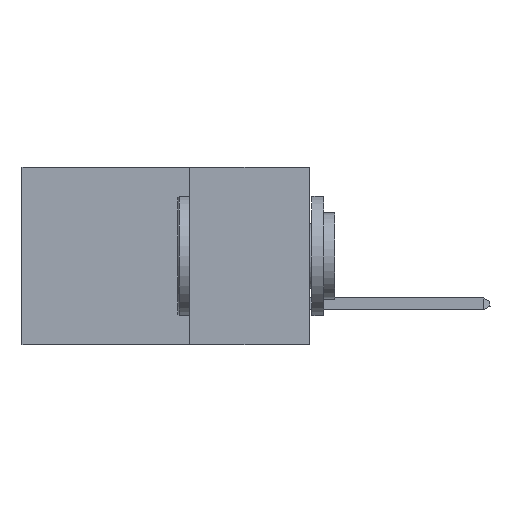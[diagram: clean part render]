
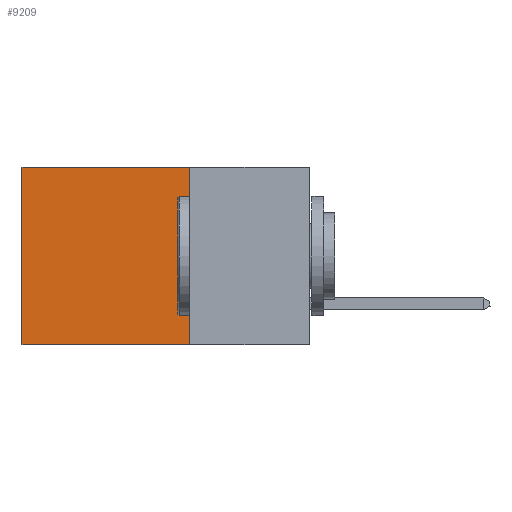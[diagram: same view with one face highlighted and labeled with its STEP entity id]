
A CAD part, left-side view. The second image highlights one B-rep face of the part: STEP entity #9209.
In plain terms, the highlighted planar face has unit normal (-1, 0, 0).
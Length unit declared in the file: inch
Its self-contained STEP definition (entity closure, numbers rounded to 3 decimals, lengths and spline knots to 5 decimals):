
#1216 = CARTESIAN_POINT ( 'NONE',  ( 0.2875, 0.25, 0. ) ) ;
#2583 = VECTOR ( 'NONE', #10977, 39.37008 ) ;
#3502 = DIRECTION ( 'NONE',  ( 1., 0., 0. ) ) ;
#3728 = DIRECTION ( 'NONE',  ( 0., 0., -1. ) ) ;
#4826 = EDGE_CURVE ( 'NONE', #24657, #20292, #8424, .T. ) ;
#4840 = VECTOR ( 'NONE', #25722, 39.37008 ) ;
#4922 = LINE ( 'NONE', #18243, #2583 ) ;
#6077 = PLANE ( 'NONE',  #7237 ) ;
#6508 = CARTESIAN_POINT ( 'NONE',  ( 0.2875, 0.6, -0.37 ) ) ;
#6531 = CARTESIAN_POINT ( 'NONE',  ( 0.2875, 0.25, 0. ) ) ;
#7147 = CARTESIAN_POINT ( 'NONE',  ( 0.2875, 0.6, 0. ) ) ;
#7237 = AXIS2_PLACEMENT_3D ( 'NONE', #25612, #3502, #3728 ) ;
#7867 = LINE ( 'NONE', #20045, #22796 ) ;
#8319 = LINE ( 'NONE', #6531, #4840 ) ;
#8424 = LINE ( 'NONE', #7147, #28677 ) ;
#9209 = ADVANCED_FACE ( 'NONE', ( #12334 ), #6077, .F. ) ;
#10647 = ORIENTED_EDGE ( 'NONE', *, *, #22903, .T. ) ;
#10977 = DIRECTION ( 'NONE',  ( 0., 1., 0. ) ) ;
#11850 = EDGE_LOOP ( 'NONE', ( #19201, #20408, #30681, #10647 ) ) ;
#12334 = FACE_OUTER_BOUND ( 'NONE', #11850, .T. ) ;
#17447 = EDGE_CURVE ( 'NONE', #26578, #20292, #4922, .T. ) ;
#18243 = CARTESIAN_POINT ( 'NONE',  ( 0.2875, 0.25, -0.37 ) ) ;
#19153 = CARTESIAN_POINT ( 'NONE',  ( 0.2875, 0.6, 0. ) ) ;
#19201 = ORIENTED_EDGE ( 'NONE', *, *, #4826, .T. ) ;
#19547 = DIRECTION ( 'NONE',  ( 0., 0., -1. ) ) ;
#19651 = VERTEX_POINT ( 'NONE', #1216 ) ;
#20045 = CARTESIAN_POINT ( 'NONE',  ( 0.2875, 0.25, 0. ) ) ;
#20292 = VERTEX_POINT ( 'NONE', #6508 ) ;
#20366 = DIRECTION ( 'NONE',  ( 0., 0., -1. ) ) ;
#20408 = ORIENTED_EDGE ( 'NONE', *, *, #17447, .F. ) ;
#22796 = VECTOR ( 'NONE', #20366, 39.37008 ) ;
#22903 = EDGE_CURVE ( 'NONE', #19651, #24657, #8319, .T. ) ;
#24657 = VERTEX_POINT ( 'NONE', #19153 ) ;
#25612 = CARTESIAN_POINT ( 'NONE',  ( 0.2875, 0.25, 0. ) ) ;
#25722 = DIRECTION ( 'NONE',  ( 0., 1., 0. ) ) ;
#26578 = VERTEX_POINT ( 'NONE', #31553 ) ;
#28677 = VECTOR ( 'NONE', #19547, 39.37008 ) ;
#29282 = EDGE_CURVE ( 'NONE', #19651, #26578, #7867, .T. ) ;
#30681 = ORIENTED_EDGE ( 'NONE', *, *, #29282, .F. ) ;
#31553 = CARTESIAN_POINT ( 'NONE',  ( 0.2875, 0.25, -0.37 ) ) ;
